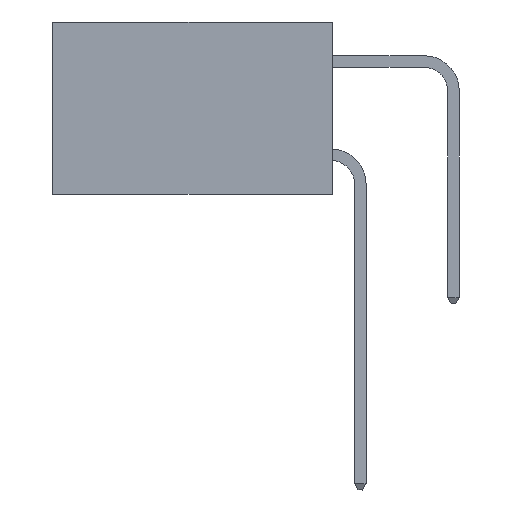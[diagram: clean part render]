
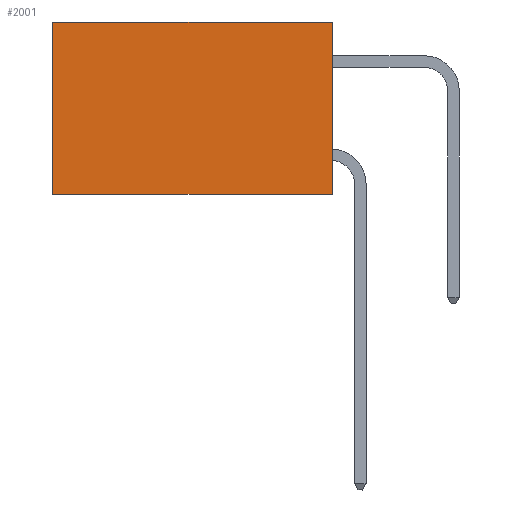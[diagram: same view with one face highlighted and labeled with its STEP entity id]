
A CAD part, left-side view. The second image highlights one B-rep face of the part: STEP entity #2001.
In plain terms, the highlighted planar face has unit normal (-1, 0, 0).
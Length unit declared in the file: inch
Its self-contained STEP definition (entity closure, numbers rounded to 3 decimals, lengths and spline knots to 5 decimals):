
#903 = DIRECTION ( 'NONE',  ( 0., 0., -1. ) ) ;
#1294 = VERTEX_POINT ( 'NONE', #26362 ) ;
#1356 = ORIENTED_EDGE ( 'NONE', *, *, #23287, .T. ) ;
#1844 = CARTESIAN_POINT ( 'NONE',  ( 0.2615, 0., -0.37 ) ) ;
#2001 = ADVANCED_FACE ( 'NONE', ( #8056 ), #24425, .F. ) ;
#2375 = LINE ( 'NONE', #1844, #24536 ) ;
#3715 = DIRECTION ( 'NONE',  ( 0., 0., -1. ) ) ;
#4496 = VERTEX_POINT ( 'NONE', #17171 ) ;
#5746 = VERTEX_POINT ( 'NONE', #6225 ) ;
#6013 = CARTESIAN_POINT ( 'NONE',  ( 0.2615, 0.6, 0. ) ) ;
#6225 = CARTESIAN_POINT ( 'NONE',  ( 0.2615, 0., -0.37 ) ) ;
#6756 = EDGE_LOOP ( 'NONE', ( #25776, #15321, #11455, #1356 ) ) ;
#8056 = FACE_OUTER_BOUND ( 'NONE', #6756, .T. ) ;
#8187 = CARTESIAN_POINT ( 'NONE',  ( 0.2615, 0., -0.37 ) ) ;
#10438 = LINE ( 'NONE', #18601, #17600 ) ;
#10972 = VERTEX_POINT ( 'NONE', #6013 ) ;
#11416 = DIRECTION ( 'NONE',  ( 0., 1., 0. ) ) ;
#11455 = ORIENTED_EDGE ( 'NONE', *, *, #16320, .F. ) ;
#11984 = VECTOR ( 'NONE', #903, 39.37008 ) ;
#15021 = VECTOR ( 'NONE', #11416, 39.37008 ) ;
#15034 = AXIS2_PLACEMENT_3D ( 'NONE', #8187, #16394, #20655 ) ;
#15321 = ORIENTED_EDGE ( 'NONE', *, *, #21949, .F. ) ;
#16320 = EDGE_CURVE ( 'NONE', #4496, #5746, #21969, .T. ) ;
#16394 = DIRECTION ( 'NONE',  ( 1., 0., 0. ) ) ;
#17171 = CARTESIAN_POINT ( 'NONE',  ( 0.2615, 0., 0. ) ) ;
#17600 = VECTOR ( 'NONE', #3715, 39.37008 ) ;
#18601 = CARTESIAN_POINT ( 'NONE',  ( 0.2615, 0.6, -0.37 ) ) ;
#19985 = LINE ( 'NONE', #20117, #15021 ) ;
#20117 = CARTESIAN_POINT ( 'NONE',  ( 0.2615, 0., 0. ) ) ;
#20655 = DIRECTION ( 'NONE',  ( 0., 0., -1. ) ) ;
#21828 = CARTESIAN_POINT ( 'NONE',  ( 0.2615, 0., -0.37 ) ) ;
#21949 = EDGE_CURVE ( 'NONE', #5746, #1294, #2375, .T. ) ;
#21969 = LINE ( 'NONE', #21828, #11984 ) ;
#23287 = EDGE_CURVE ( 'NONE', #4496, #10972, #19985, .T. ) ;
#23933 = EDGE_CURVE ( 'NONE', #10972, #1294, #10438, .T. ) ;
#24425 = PLANE ( 'NONE',  #15034 ) ;
#24536 = VECTOR ( 'NONE', #24794, 39.37008 ) ;
#24794 = DIRECTION ( 'NONE',  ( 0., 1., 0. ) ) ;
#25776 = ORIENTED_EDGE ( 'NONE', *, *, #23933, .T. ) ;
#26362 = CARTESIAN_POINT ( 'NONE',  ( 0.2615, 0.6, -0.37 ) ) ;
